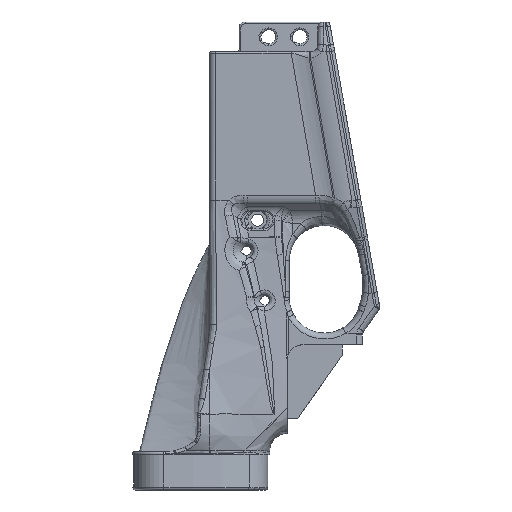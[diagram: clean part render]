
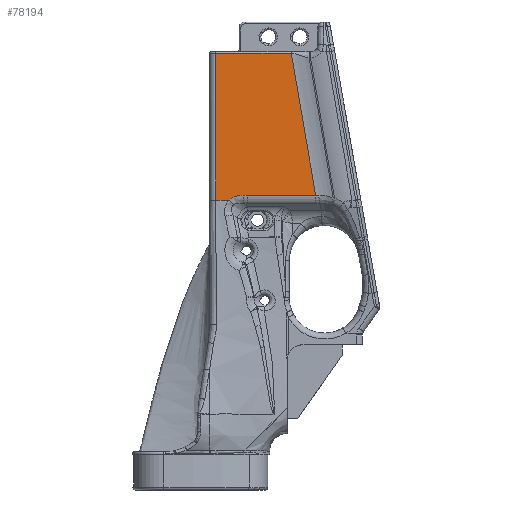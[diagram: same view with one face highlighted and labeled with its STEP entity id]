
A CAD part, left-side view. The second image highlights one B-rep face of the part: STEP entity #78194.
In plain terms, the highlighted planar face has unit normal (-1, 0, 0).
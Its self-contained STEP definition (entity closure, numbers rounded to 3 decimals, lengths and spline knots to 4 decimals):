
#945 = ORIENTED_EDGE ( 'NONE', *, *, #106932, .F. ) ;
#5482 = CARTESIAN_POINT ( 'NONE',  ( -0.7, -0.3753, 3.6638 ) ) ;
#6571 = CARTESIAN_POINT ( 'NONE',  ( -0.7, -0.4657, 3.7008 ) ) ;
#6880 = DIRECTION ( 'NONE',  ( 0., 0., 1. ) ) ;
#7946 = CARTESIAN_POINT ( 'NONE',  ( -0.7, -2.8877, 6.15 ) ) ;
#9411 = B_SPLINE_CURVE_WITH_KNOTS ( 'NONE', 3,
 ( #62664, #36163, #11407, #61036 ),
 .UNSPECIFIED., .F., .F.,
 ( 4, 4 ),
 ( 0.64, 0.8438 ),
 .UNSPECIFIED. ) ;
#10895 = EDGE_CURVE ( 'NONE', #83763, #46964, #47436, .T. ) ;
#11407 = CARTESIAN_POINT ( 'NONE',  ( -0.7, -0.1435, 3.63 ) ) ;
#11953 = CARTESIAN_POINT ( 'NONE',  ( -0.7, -0.3267, 3.63 ) ) ;
#12459 = CARTESIAN_POINT ( 'NONE',  ( -0.7, -0.5738, 3.7128 ) ) ;
#14347 = EDGE_CURVE ( 'NONE', #62709, #83763, #101929, .T. ) ;
#15955 = EDGE_CURVE ( 'NONE', #39047, #62709, #77031, .T. ) ;
#16136 = CARTESIAN_POINT ( 'NONE',  ( -0.7, -2.8877, 3.7128 ) ) ;
#18597 = DIRECTION ( 'NONE',  ( 0., 0.169, 0.986 ) ) ;
#21187 = EDGE_CURVE ( 'NONE', #99523, #46964, #9411, .T. ) ;
#27509 = CARTESIAN_POINT ( 'NONE',  ( -0.7, -0.2304, 3.63 ) ) ;
#28260 = CARTESIAN_POINT ( 'NONE',  ( -0.7, -0.5518, 3.7128 ) ) ;
#36163 = CARTESIAN_POINT ( 'NONE',  ( -0.7, -0.1869, 3.63 ) ) ;
#36839 = CARTESIAN_POINT ( 'NONE',  ( -0.7, -0.2875, 3.63 ) ) ;
#36989 = VERTEX_POINT ( 'NONE', #95214 ) ;
#38855 = CARTESIAN_POINT ( 'NONE',  ( -0.7, -0.316, 3.63 ) ) ;
#39047 = VERTEX_POINT ( 'NONE', #97154 ) ;
#39048 = CARTESIAN_POINT ( 'NONE',  ( -0.7, -0.4037, 3.6799 ) ) ;
#40178 = LINE ( 'NONE', #90903, #93080 ) ;
#42464 = VERTEX_POINT ( 'NONE', #107869 ) ;
#45532 = CARTESIAN_POINT ( 'NONE',  ( -0.7, -0.3321, 3.63 ) ) ;
#46001 = ORIENTED_EDGE ( 'NONE', *, *, #15955, .T. ) ;
#46964 = VERTEX_POINT ( 'NONE', #57015 ) ;
#47436 = B_SPLINE_CURVE_WITH_KNOTS ( 'NONE', 3,
 ( #69475, #104181, #103633, #61764 ),
 .UNSPECIFIED., .F., .F.,
 ( 4, 4 ),
 ( -0.1525, -0.0893 ),
 .UNSPECIFIED. ) ;
#47890 = CARTESIAN_POINT ( 'NONE',  ( -0.7, -0.366, 3.6578 ) ) ;
#48964 = CARTESIAN_POINT ( 'NONE',  ( -0.7, -0.4551, 3.698 ) ) ;
#49612 = ORIENTED_EDGE ( 'NONE', *, *, #52403, .T. ) ;
#51197 = DIRECTION ( 'NONE',  ( 0., 1., 0. ) ) ;
#52403 = EDGE_CURVE ( 'NONE', #98588, #36989, #55587, .T. ) ;
#52758 = CARTESIAN_POINT ( 'NONE',  ( -0.7, -1.4229, 5.8986 ) ) ;
#53247 = ORIENTED_EDGE ( 'NONE', *, *, #10895, .T. ) ;
#53825 = CARTESIAN_POINT ( 'NONE',  ( -0.7, -0.3214, 3.63 ) ) ;
#55587 = B_SPLINE_CURVE_WITH_KNOTS ( 'NONE', 3,
 ( #38855, #53825, #11953, #45532 ),
 .UNSPECIFIED., .F., .F.,
 ( 4, 4 ),
 ( 0., 0.0855 ),
 .UNSPECIFIED. ) ;
#55642 = CARTESIAN_POINT ( 'NONE',  ( -0.7, -0.3321, 3.63 ) ) ;
#55808 = VECTOR ( 'NONE', #51197, 39.3701 ) ;
#56428 = B_SPLINE_CURVE_WITH_KNOTS ( 'NONE', 3,
 ( #55642, #82066, #89255, #47890, #5482, #39048, #61902, #48964, #6571, #103781, #90315, #89797, #28260, #73809 ),
 .UNSPECIFIED., .F., .F.,
 ( 4, 2, 2, 2, 2, 2, 4 ),
 ( 0., 0.0008, 0.0017, 0.0033, 0.0042, 0.005, 0.0067 ),
 .UNSPECIFIED. ) ;
#56831 = ORIENTED_EDGE ( 'NONE', *, *, #97205, .T. ) ;
#57015 = CARTESIAN_POINT ( 'NONE',  ( -0.7, -0.1, 3.63 ) ) ;
#58992 = EDGE_LOOP ( 'NONE', ( #49612, #63902, #88911, #56831, #46001, #94645, #53247, #105114, #945 ) ) ;
#61036 = CARTESIAN_POINT ( 'NONE',  ( -0.7, -0.1, 3.63 ) ) ;
#61764 = CARTESIAN_POINT ( 'NONE',  ( -0.7, -0.1, 3.63 ) ) ;
#61902 = CARTESIAN_POINT ( 'NONE',  ( -0.7, -0.4238, 3.6883 ) ) ;
#62664 = CARTESIAN_POINT ( 'NONE',  ( -0.7, -0.2304, 3.63 ) ) ;
#62709 = VERTEX_POINT ( 'NONE', #67630 ) ;
#63694 = FACE_OUTER_BOUND ( 'NONE', #58992, .T. ) ;
#63902 = ORIENTED_EDGE ( 'NONE', *, *, #94831, .T. ) ;
#65126 = VECTOR ( 'NONE', #99924, 39.3701 ) ;
#65260 = LINE ( 'NONE', #16136, #65126 ) ;
#66949 = DIRECTION ( 'NONE',  ( -1., 0., 0. ) ) ;
#67238 = CARTESIAN_POINT ( 'NONE',  ( -0.7, 0., 6.12 ) ) ;
#67630 = CARTESIAN_POINT ( 'NONE',  ( -0.7, -1.3849, 6.12 ) ) ;
#69475 = CARTESIAN_POINT ( 'NONE',  ( -0.7, -0.1, 6.12 ) ) ;
#73121 = VERTEX_POINT ( 'NONE', #12459 ) ;
#73809 = CARTESIAN_POINT ( 'NONE',  ( -0.7, -0.5738, 3.7128 ) ) ;
#77031 = LINE ( 'NONE', #52758, #97917 ) ;
#78194 = ADVANCED_FACE ( 'NONE', ( #63694 ), #97842, .T. ) ;
#78230 = CARTESIAN_POINT ( 'NONE',  ( -0.7, -0.259, 3.63 ) ) ;
#79721 = CARTESIAN_POINT ( 'NONE',  ( -0.7, -0.316, 3.63 ) ) ;
#81518 = AXIS2_PLACEMENT_3D ( 'NONE', #7946, #66949, #6880 ) ;
#82066 = CARTESIAN_POINT ( 'NONE',  ( -0.7, -0.34, 3.6377 ) ) ;
#83763 = VERTEX_POINT ( 'NONE', #100637 ) ;
#88822 = CARTESIAN_POINT ( 'NONE',  ( -0.7, -0.2304, 3.63 ) ) ;
#88911 = ORIENTED_EDGE ( 'NONE', *, *, #92866, .T. ) ;
#89255 = CARTESIAN_POINT ( 'NONE',  ( -0.7, -0.3483, 3.6447 ) ) ;
#89797 = CARTESIAN_POINT ( 'NONE',  ( -0.7, -0.5301, 3.7116 ) ) ;
#90315 = CARTESIAN_POINT ( 'NONE',  ( -0.7, -0.4978, 3.7072 ) ) ;
#90903 = CARTESIAN_POINT ( 'NONE',  ( -0.7, -2.8877, 3.7128 ) ) ;
#92866 = EDGE_CURVE ( 'NONE', #73121, #42464, #40178, .T. ) ;
#93080 = VECTOR ( 'NONE', #108524, 39.3701 ) ;
#94645 = ORIENTED_EDGE ( 'NONE', *, *, #14347, .T. ) ;
#94831 = EDGE_CURVE ( 'NONE', #36989, #73121, #56428, .T. ) ;
#95214 = CARTESIAN_POINT ( 'NONE',  ( -0.7, -0.3321, 3.63 ) ) ;
#95860 = CARTESIAN_POINT ( 'NONE',  ( -0.7, -0.316, 3.63 ) ) ;
#97154 = CARTESIAN_POINT ( 'NONE',  ( -0.7, -1.798, 3.7128 ) ) ;
#97205 = EDGE_CURVE ( 'NONE', #42464, #39047, #65260, .T. ) ;
#97842 = PLANE ( 'NONE',  #81518 ) ;
#97917 = VECTOR ( 'NONE', #18597, 39.3701 ) ;
#98588 = VERTEX_POINT ( 'NONE', #79721 ) ;
#99523 = VERTEX_POINT ( 'NONE', #88822 ) ;
#99924 = DIRECTION ( 'NONE',  ( 0., -1., 0. ) ) ;
#100637 = CARTESIAN_POINT ( 'NONE',  ( -0.7, -0.1, 6.12 ) ) ;
#101929 = LINE ( 'NONE', #67238, #55808 ) ;
#103633 = CARTESIAN_POINT ( 'NONE',  ( -0.7, -0.1, 4.46 ) ) ;
#103781 = CARTESIAN_POINT ( 'NONE',  ( -0.7, -0.4871, 3.7054 ) ) ;
#104181 = CARTESIAN_POINT ( 'NONE',  ( -0.7, -0.1, 5.29 ) ) ;
#105114 = ORIENTED_EDGE ( 'NONE', *, *, #21187, .F. ) ;
#106932 = EDGE_CURVE ( 'NONE', #98588, #99523, #107378, .T. ) ;
#107378 = B_SPLINE_CURVE_WITH_KNOTS ( 'NONE', 3,
 ( #95860, #36839, #78230, #27509 ),
 .UNSPECIFIED., .F., .F.,
 ( 4, 4 ),
 ( 0.5062, 0.64 ),
 .UNSPECIFIED. ) ;
#107869 = CARTESIAN_POINT ( 'NONE',  ( -0.7, -0.64, 3.7128 ) ) ;
#108524 = DIRECTION ( 'NONE',  ( 0., -1., 0. ) ) ;
